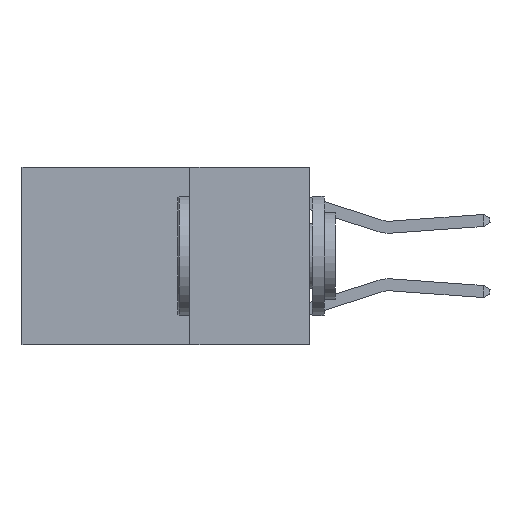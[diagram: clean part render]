
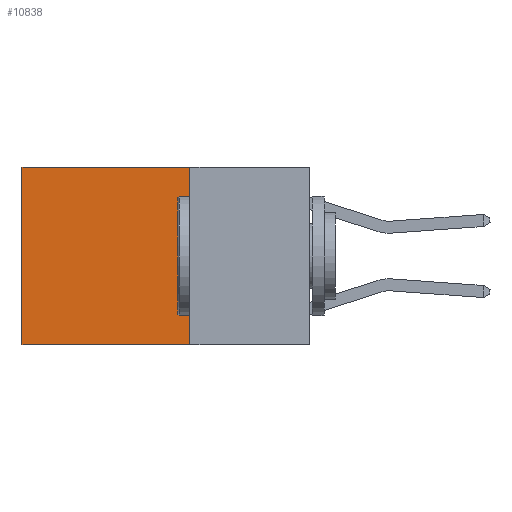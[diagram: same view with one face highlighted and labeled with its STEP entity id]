
A CAD part, left-side view. The second image highlights one B-rep face of the part: STEP entity #10838.
In plain terms, the highlighted planar face has unit normal (-1, 0, 0).
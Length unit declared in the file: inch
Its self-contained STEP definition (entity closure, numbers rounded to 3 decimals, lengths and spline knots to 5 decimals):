
#78 = EDGE_CURVE ( 'NONE', #1829, #19624, #11538, .T. ) ;
#750 = CARTESIAN_POINT ( 'NONE',  ( 0.2625, 0.6, 0. ) ) ;
#832 = CARTESIAN_POINT ( 'NONE',  ( 0.2625, 0.25, 0. ) ) ;
#851 = LINE ( 'NONE', #2701, #870 ) ;
#870 = VECTOR ( 'NONE', #18960, 39.37008 ) ;
#1037 = ORIENTED_EDGE ( 'NONE', *, *, #2387, .F. ) ;
#1829 = VERTEX_POINT ( 'NONE', #11514 ) ;
#2387 = EDGE_CURVE ( 'NONE', #3452, #21136, #11084, .T. ) ;
#2701 = CARTESIAN_POINT ( 'NONE',  ( 0.2625, 0.25, -0.37 ) ) ;
#3306 = DIRECTION ( 'NONE',  ( 1., 0., 0. ) ) ;
#3452 = VERTEX_POINT ( 'NONE', #19096 ) ;
#3765 = EDGE_CURVE ( 'NONE', #21136, #19624, #851, .T. ) ;
#5045 = ORIENTED_EDGE ( 'NONE', *, *, #7571, .T. ) ;
#5631 = VECTOR ( 'NONE', #19774, 39.37008 ) ;
#7377 = DIRECTION ( 'NONE',  ( 0., 0., -1. ) ) ;
#7571 = EDGE_CURVE ( 'NONE', #3452, #1829, #9662, .T. ) ;
#8251 = VECTOR ( 'NONE', #7377, 39.37008 ) ;
#9662 = LINE ( 'NONE', #832, #5631 ) ;
#9703 = CARTESIAN_POINT ( 'NONE',  ( 0.2625, 0.25, 0. ) ) ;
#10838 = ADVANCED_FACE ( 'NONE', ( #13195 ), #20259, .F. ) ;
#11084 = LINE ( 'NONE', #21749, #8251 ) ;
#11216 = VECTOR ( 'NONE', #18623, 39.37008 ) ;
#11514 = CARTESIAN_POINT ( 'NONE',  ( 0.2625, 0.6, 0. ) ) ;
#11538 = LINE ( 'NONE', #750, #11216 ) ;
#11958 = ORIENTED_EDGE ( 'NONE', *, *, #78, .T. ) ;
#13195 = FACE_OUTER_BOUND ( 'NONE', #20024, .T. ) ;
#14268 = AXIS2_PLACEMENT_3D ( 'NONE', #9703, #3306, #19215 ) ;
#15989 = CARTESIAN_POINT ( 'NONE',  ( 0.2625, 0.25, -0.37 ) ) ;
#18623 = DIRECTION ( 'NONE',  ( 0., 0., -1. ) ) ;
#18960 = DIRECTION ( 'NONE',  ( 0., 1., 0. ) ) ;
#19096 = CARTESIAN_POINT ( 'NONE',  ( 0.2625, 0.25, 0. ) ) ;
#19119 = CARTESIAN_POINT ( 'NONE',  ( 0.2625, 0.6, -0.37 ) ) ;
#19215 = DIRECTION ( 'NONE',  ( 0., 0., -1. ) ) ;
#19624 = VERTEX_POINT ( 'NONE', #19119 ) ;
#19774 = DIRECTION ( 'NONE',  ( 0., 1., 0. ) ) ;
#20024 = EDGE_LOOP ( 'NONE', ( #11958, #22823, #1037, #5045 ) ) ;
#20259 = PLANE ( 'NONE',  #14268 ) ;
#21136 = VERTEX_POINT ( 'NONE', #15989 ) ;
#21749 = CARTESIAN_POINT ( 'NONE',  ( 0.2625, 0.25, 0. ) ) ;
#22823 = ORIENTED_EDGE ( 'NONE', *, *, #3765, .F. ) ;
